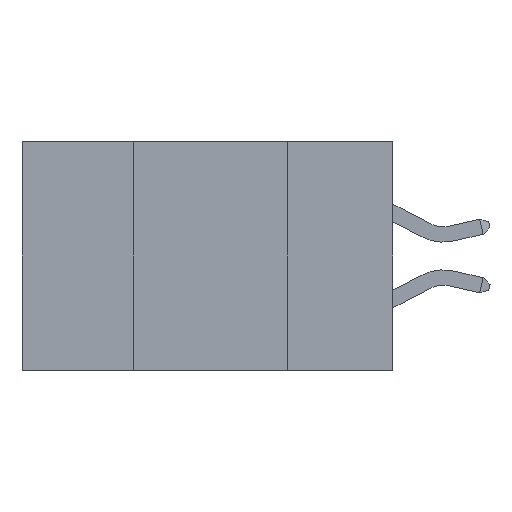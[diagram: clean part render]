
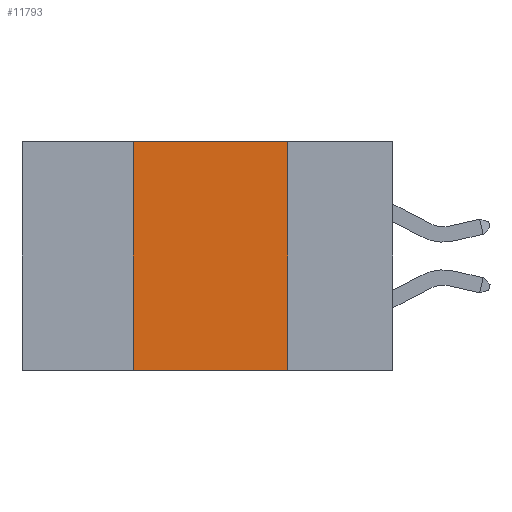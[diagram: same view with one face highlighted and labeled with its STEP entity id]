
A CAD part, left-side view. The second image highlights one B-rep face of the part: STEP entity #11793.
In plain terms, the highlighted planar face has unit normal (-1, 0, 0).
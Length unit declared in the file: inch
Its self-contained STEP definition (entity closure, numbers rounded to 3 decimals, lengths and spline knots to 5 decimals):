
#135 = CARTESIAN_POINT ( 'NONE',  ( 0., 0.6, 0. ) ) ;
#417 = VERTEX_POINT ( 'NONE', #8340 ) ;
#1955 = VERTEX_POINT ( 'NONE', #6975 ) ;
#2636 = VERTEX_POINT ( 'NONE', #4277 ) ;
#2678 = LINE ( 'NONE', #19162, #3626 ) ;
#3042 = DIRECTION ( 'NONE',  ( 1., 0., 0. ) ) ;
#3093 = CARTESIAN_POINT ( 'NONE',  ( 0., 0.42, 0. ) ) ;
#3527 = CARTESIAN_POINT ( 'NONE',  ( 0., 0.6, -0.37 ) ) ;
#3626 = VECTOR ( 'NONE', #17407, 39.37008 ) ;
#3812 = VECTOR ( 'NONE', #10935, 39.37008 ) ;
#4277 = CARTESIAN_POINT ( 'NONE',  ( 0., 0.17, 0. ) ) ;
#4627 = PLANE ( 'NONE',  #6667 ) ;
#6209 = DIRECTION ( 'NONE',  ( 0., 0., 1. ) ) ;
#6667 = AXIS2_PLACEMENT_3D ( 'NONE', #135, #3042, #15104 ) ;
#6975 = CARTESIAN_POINT ( 'NONE',  ( 0., 0.42, 0. ) ) ;
#7388 = LINE ( 'NONE', #3527, #3812 ) ;
#7718 = EDGE_CURVE ( 'NONE', #13974, #417, #7388, .T. ) ;
#7958 = ORIENTED_EDGE ( 'NONE', *, *, #15896, .F. ) ;
#8340 = CARTESIAN_POINT ( 'NONE',  ( 0., 0.17, -0.37 ) ) ;
#9188 = ORIENTED_EDGE ( 'NONE', *, *, #10796, .F. ) ;
#9360 = CARTESIAN_POINT ( 'NONE',  ( 0., 0.17, 0. ) ) ;
#9402 = EDGE_LOOP ( 'NONE', ( #7958, #9188, #18710, #10296 ) ) ;
#10296 = ORIENTED_EDGE ( 'NONE', *, *, #7718, .T. ) ;
#10757 = DIRECTION ( 'NONE',  ( 0., 0., -1. ) ) ;
#10796 = EDGE_CURVE ( 'NONE', #1955, #2636, #2678, .T. ) ;
#10935 = DIRECTION ( 'NONE',  ( 0., -1., 0. ) ) ;
#11793 = ADVANCED_FACE ( 'NONE', ( #15618 ), #4627, .F. ) ;
#12223 = VECTOR ( 'NONE', #6209, 39.37008 ) ;
#13974 = VERTEX_POINT ( 'NONE', #18759 ) ;
#15104 = DIRECTION ( 'NONE',  ( 0., 0., -1. ) ) ;
#15618 = FACE_OUTER_BOUND ( 'NONE', #9402, .T. ) ;
#15896 = EDGE_CURVE ( 'NONE', #2636, #417, #19125, .T. ) ;
#16299 = VECTOR ( 'NONE', #10757, 39.37008 ) ;
#17407 = DIRECTION ( 'NONE',  ( 0., -1., 0. ) ) ;
#17427 = LINE ( 'NONE', #3093, #12223 ) ;
#17707 = EDGE_CURVE ( 'NONE', #13974, #1955, #17427, .T. ) ;
#18710 = ORIENTED_EDGE ( 'NONE', *, *, #17707, .F. ) ;
#18759 = CARTESIAN_POINT ( 'NONE',  ( 0., 0.42, -0.37 ) ) ;
#19125 = LINE ( 'NONE', #9360, #16299 ) ;
#19162 = CARTESIAN_POINT ( 'NONE',  ( 0., 0.6, 0. ) ) ;
